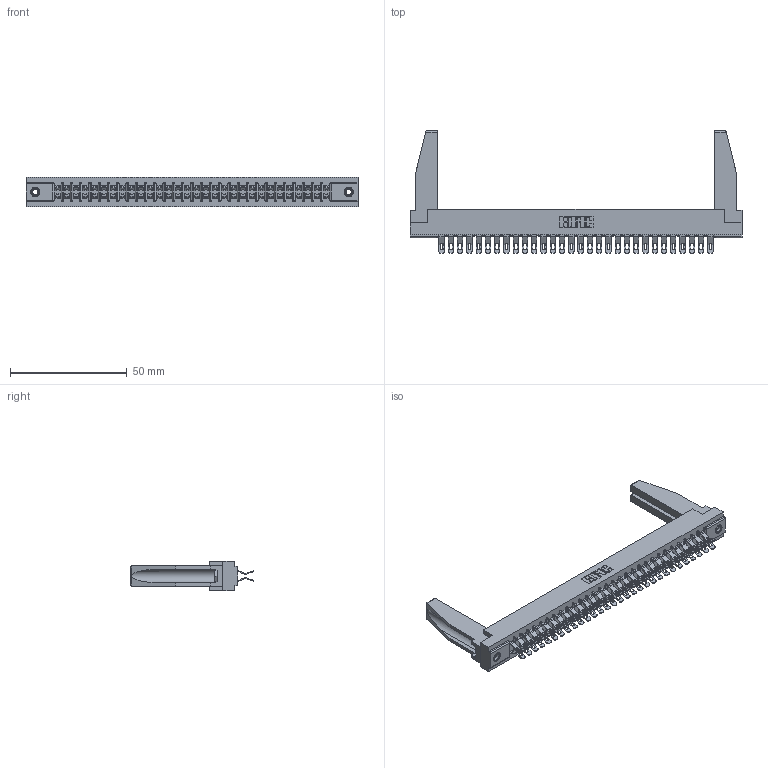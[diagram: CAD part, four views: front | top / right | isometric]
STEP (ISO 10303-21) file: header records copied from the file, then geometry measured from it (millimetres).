
FILE_DESCRIPTION (( 'STEP AP203' ), '1' );
FILE_NAME ('357-060-455-278.STEP', '2020-10-04T13:51:33', ( '' ), ( '' ), 'SwSTEP 2.0', 'SolidWorks 2020', '' );
FILE_SCHEMA (( 'CONFIG_CONTROL_DESIGN' ));
Length unit declared in the file: inch
Products named in the file (5): 345-250-001_345-250-001-102; 307 Part_.156 Dia Mounting Holes; 307-290-001_555; 307-220-078; 357-060-455-278
Assembly tree (65 placements, depth 2):
  357-060-455-278
    307 Part_.156 Dia Mounting Holes
    307-290-001_555  x60
    307-220-078  x2
    345-250-001_345-250-001-102  x2
Bounding box: 141.88 x 52.45 x 12.7 mm (x, y, z)
Volume: 19174.8 mm3; surface area: 23151.9 mm2
Topology: 65 solids, 65 shells, 3939 faces, 11513 edges, 7502 vertices
Faces by surface type: plane 2194, cylinder 1667, sphere 62, cone 12, torus 4
Entity records: 31134 total; most frequent: CARTESIAN_POINT 5112, ORIENTED_EDGE 5026, DIRECTION 4973, EDGE_CURVE 2513, LINE 1915, VECTOR 1915, VERTEX_POINT 1626, AXIS2_PLACEMENT_3D 1529
